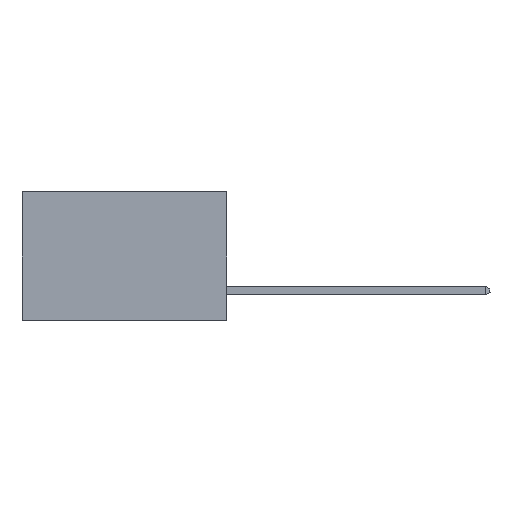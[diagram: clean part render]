
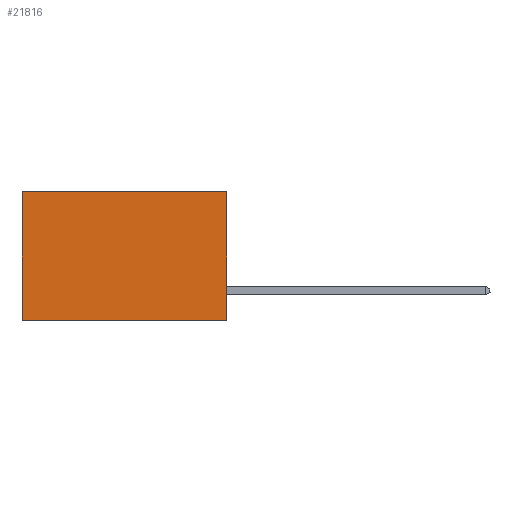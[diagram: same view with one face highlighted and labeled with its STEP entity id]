
A CAD part, left-side view. The second image highlights one B-rep face of the part: STEP entity #21816.
In plain terms, the highlighted planar face has unit normal (-1, 0, 0).
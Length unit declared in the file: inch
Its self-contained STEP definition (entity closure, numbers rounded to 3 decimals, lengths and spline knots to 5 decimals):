
#1454 = VERTEX_POINT ( 'NONE', #3422 ) ;
#1775 = VERTEX_POINT ( 'NONE', #15436 ) ;
#2420 = EDGE_CURVE ( 'NONE', #19065, #1775, #21301, .T. ) ;
#2798 = DIRECTION ( 'NONE',  ( 0., 1., 0. ) ) ;
#3422 = CARTESIAN_POINT ( 'NONE',  ( 0.277, 0.59, -0.37 ) ) ;
#3632 = DIRECTION ( 'NONE',  ( 0., 0., -1. ) ) ;
#3814 = CARTESIAN_POINT ( 'NONE',  ( 0.277, 0., -0.37 ) ) ;
#4530 = AXIS2_PLACEMENT_3D ( 'NONE', #3814, #6008, #20311 ) ;
#5586 = DIRECTION ( 'NONE',  ( 0., 0., -1. ) ) ;
#6008 = DIRECTION ( 'NONE',  ( 1., 0., 0. ) ) ;
#6637 = ORIENTED_EDGE ( 'NONE', *, *, #18913, .T. ) ;
#7634 = VECTOR ( 'NONE', #5586, 39.37008 ) ;
#8928 = VERTEX_POINT ( 'NONE', #16301 ) ;
#9201 = VECTOR ( 'NONE', #2798, 39.37008 ) ;
#10376 = FACE_OUTER_BOUND ( 'NONE', #17605, .T. ) ;
#10423 = ORIENTED_EDGE ( 'NONE', *, *, #24987, .F. ) ;
#10598 = ORIENTED_EDGE ( 'NONE', *, *, #14330, .F. ) ;
#12191 = CARTESIAN_POINT ( 'NONE',  ( 0.277, 0., 0. ) ) ;
#13345 = ORIENTED_EDGE ( 'NONE', *, *, #2420, .T. ) ;
#13558 = VECTOR ( 'NONE', #3632, 39.37008 ) ;
#14330 = EDGE_CURVE ( 'NONE', #19065, #8928, #18977, .T. ) ;
#15072 = CARTESIAN_POINT ( 'NONE',  ( 0.277, 0., -0.37 ) ) ;
#15436 = CARTESIAN_POINT ( 'NONE',  ( 0.277, 0.59, 0. ) ) ;
#15801 = VECTOR ( 'NONE', #20309, 39.37008 ) ;
#16301 = CARTESIAN_POINT ( 'NONE',  ( 0.277, 0., -0.37 ) ) ;
#16561 = CARTESIAN_POINT ( 'NONE',  ( 0.277, 0., 0. ) ) ;
#17605 = EDGE_LOOP ( 'NONE', ( #6637, #10423, #10598, #13345 ) ) ;
#17891 = CARTESIAN_POINT ( 'NONE',  ( 0.277, 0., -0.37 ) ) ;
#18247 = PLANE ( 'NONE',  #4530 ) ;
#18913 = EDGE_CURVE ( 'NONE', #1775, #1454, #24615, .T. ) ;
#18977 = LINE ( 'NONE', #17891, #13558 ) ;
#19065 = VERTEX_POINT ( 'NONE', #12191 ) ;
#20309 = DIRECTION ( 'NONE',  ( 0., 1., 0. ) ) ;
#20311 = DIRECTION ( 'NONE',  ( 0., 0., -1. ) ) ;
#21301 = LINE ( 'NONE', #16561, #15801 ) ;
#21816 = ADVANCED_FACE ( 'NONE', ( #10376 ), #18247, .F. ) ;
#24615 = LINE ( 'NONE', #26036, #7634 ) ;
#24893 = LINE ( 'NONE', #15072, #9201 ) ;
#24987 = EDGE_CURVE ( 'NONE', #8928, #1454, #24893, .T. ) ;
#26036 = CARTESIAN_POINT ( 'NONE',  ( 0.277, 0.59, -0.37 ) ) ;
